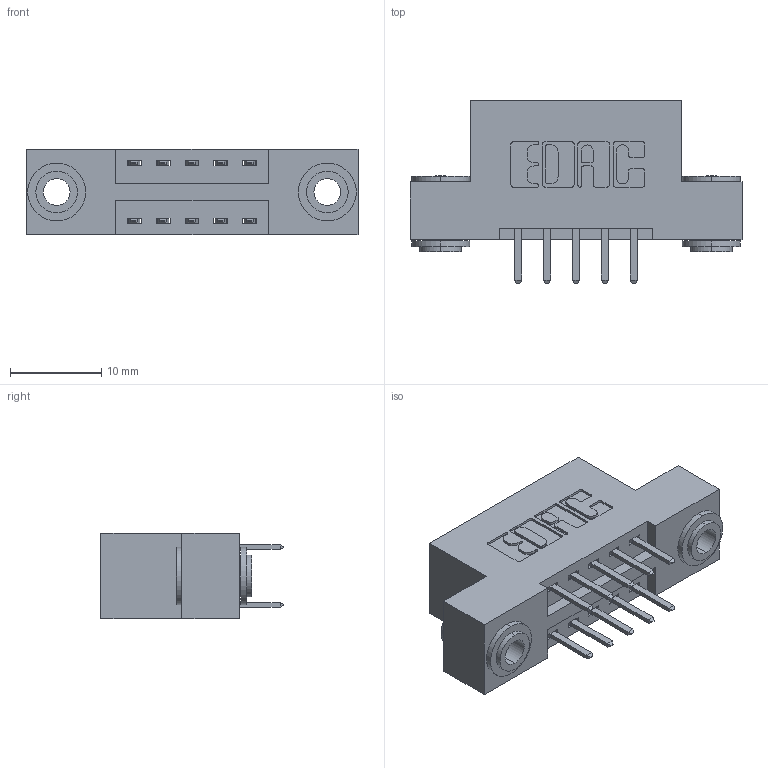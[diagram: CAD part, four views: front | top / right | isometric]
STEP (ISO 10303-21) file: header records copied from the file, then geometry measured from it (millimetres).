
FILE_DESCRIPTION (( 'STEP AP203' ), '1' );
FILE_NAME ('396-010-520-203.STEP', '2019-10-29T18:37:51', ( '' ), ( '' ), 'SwSTEP 2.0', 'SolidWorks 2016', '' );
FILE_SCHEMA (( 'CONFIG_CONTROL_DESIGN' ));
Length unit declared in the file: inch
Products named in the file (4): 345-250-002_345-250-002-102; 345-292-001_345-293-120; 346 Part_Flush Mounting Lugs - 0.156 Dia-TH; 396-010-520-203
Assembly tree (13 placements, depth 2):
  396-010-520-203
    346 Part_Flush Mounting Lugs - 0.156 Dia-TH
    345-292-001_345-293-120  x10
    345-250-002_345-250-002-102  x2
Bounding box: 36.45 x 20.02 x 9.4 mm (x, y, z)
Volume: 3281.9 mm3; surface area: 4133.5 mm2
Topology: 13 solids, 13 shells, 720 faces, 2035 edges, 1326 vertices
Faces by surface type: plane 456, cylinder 256, cone 8
Entity records: 9008 total; most frequent: CARTESIAN_POINT 1523, ORIENTED_EDGE 1438, DIRECTION 1413, EDGE_CURVE 719, LINE 539, VECTOR 539, VERTEX_POINT 474, AXIS2_PLACEMENT_3D 437
